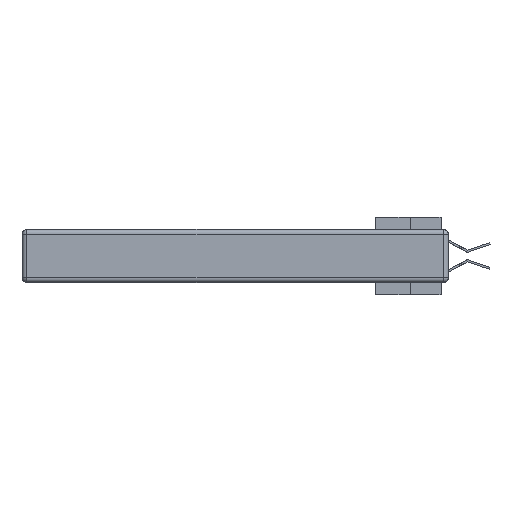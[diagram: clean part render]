
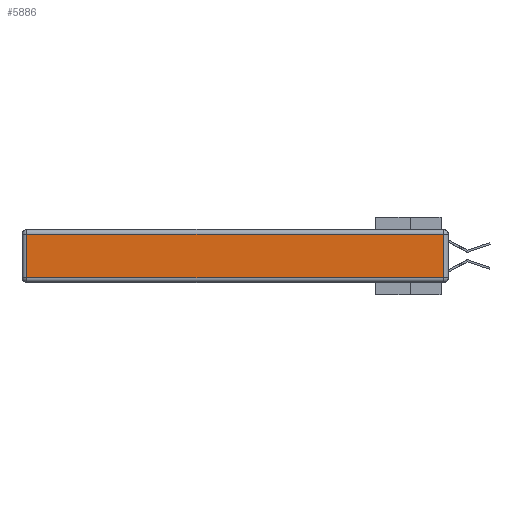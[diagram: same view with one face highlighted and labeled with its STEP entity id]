
A CAD part, left-side view. The second image highlights one B-rep face of the part: STEP entity #5886.
In plain terms, the highlighted planar face has unit normal (-1, 0, 0).
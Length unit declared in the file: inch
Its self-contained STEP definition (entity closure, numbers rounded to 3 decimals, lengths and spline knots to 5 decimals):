
#1101 = VECTOR ( 'NONE', #33465, 39.37008 ) ;
#2591 = PLANE ( 'NONE',  #11049 ) ;
#2991 = DIRECTION ( 'NONE',  ( 0., 0., 1. ) ) ;
#3303 = VECTOR ( 'NONE', #29326, 39.37008 ) ;
#3625 = ORIENTED_EDGE ( 'NONE', *, *, #7788, .T. ) ;
#3788 = ORIENTED_EDGE ( 'NONE', *, *, #15787, .T. ) ;
#4212 = CARTESIAN_POINT ( 'NONE',  ( 0., 2.72, -0.313 ) ) ;
#5886 = ADVANCED_FACE ( 'NONE', ( #37871 ), #2591, .T. ) ;
#6214 = DIRECTION ( 'NONE',  ( 0., 0., 1. ) ) ;
#7788 = EDGE_CURVE ( 'NONE', #18891, #15720, #30011, .T. ) ;
#8386 = DIRECTION ( 'NONE',  ( 0., 1., 0. ) ) ;
#8896 = CARTESIAN_POINT ( 'NONE',  ( 0., 2.72, -0.03 ) ) ;
#10625 = VECTOR ( 'NONE', #6214, 39.37008 ) ;
#11049 = AXIS2_PLACEMENT_3D ( 'NONE', #33846, #30361, #2991 ) ;
#15404 = VERTEX_POINT ( 'NONE', #8896 ) ;
#15720 = VERTEX_POINT ( 'NONE', #16662 ) ;
#15787 = EDGE_CURVE ( 'NONE', #15404, #18891, #20676, .T. ) ;
#16662 = CARTESIAN_POINT ( 'NONE',  ( 0., 0.03, -0.313 ) ) ;
#18891 = VERTEX_POINT ( 'NONE', #4212 ) ;
#19050 = EDGE_CURVE ( 'NONE', #23185, #15404, #26682, .T. ) ;
#20676 = LINE ( 'NONE', #22977, #3303 ) ;
#22977 = CARTESIAN_POINT ( 'NONE',  ( 0., 2.72, -0.343 ) ) ;
#23185 = VERTEX_POINT ( 'NONE', #23872 ) ;
#23622 = LINE ( 'NONE', #24504, #10625 ) ;
#23852 = ORIENTED_EDGE ( 'NONE', *, *, #35443, .T. ) ;
#23872 = CARTESIAN_POINT ( 'NONE',  ( 0., 0.03, -0.03 ) ) ;
#24504 = CARTESIAN_POINT ( 'NONE',  ( 0., 0.03, -0.343 ) ) ;
#24574 = EDGE_LOOP ( 'NONE', ( #3625, #23852, #37213, #3788 ) ) ;
#26682 = LINE ( 'NONE', #32627, #38228 ) ;
#29326 = DIRECTION ( 'NONE',  ( 0., 0., -1. ) ) ;
#30011 = LINE ( 'NONE', #36164, #1101 ) ;
#30361 = DIRECTION ( 'NONE',  ( -1., 0., 0. ) ) ;
#32627 = CARTESIAN_POINT ( 'NONE',  ( 0., 2.75, -0.03 ) ) ;
#33465 = DIRECTION ( 'NONE',  ( 0., -1., 0. ) ) ;
#33846 = CARTESIAN_POINT ( 'NONE',  ( 0., 0., -0.343 ) ) ;
#35443 = EDGE_CURVE ( 'NONE', #15720, #23185, #23622, .T. ) ;
#36164 = CARTESIAN_POINT ( 'NONE',  ( 0., 0., -0.313 ) ) ;
#37213 = ORIENTED_EDGE ( 'NONE', *, *, #19050, .T. ) ;
#37871 = FACE_OUTER_BOUND ( 'NONE', #24574, .T. ) ;
#38228 = VECTOR ( 'NONE', #8386, 39.37008 ) ;
